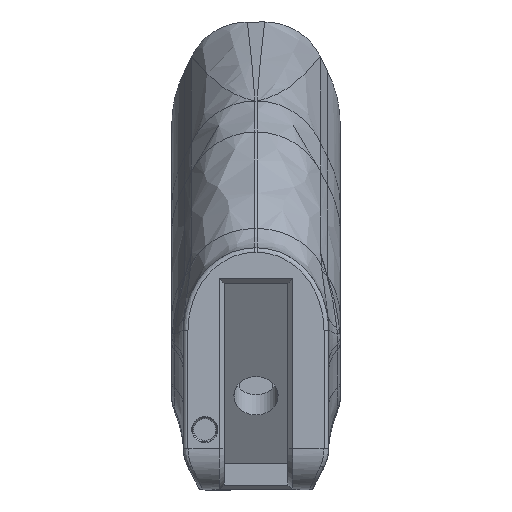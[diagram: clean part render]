
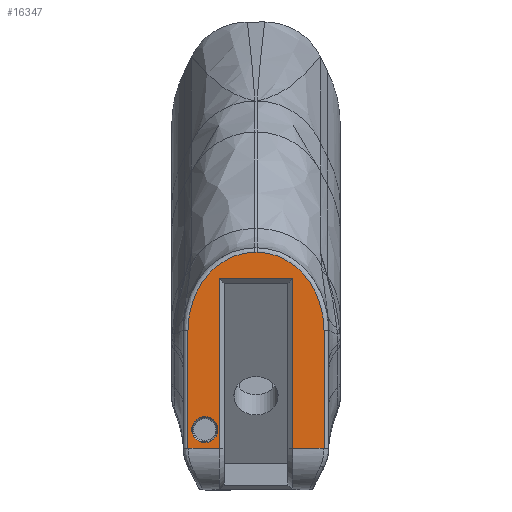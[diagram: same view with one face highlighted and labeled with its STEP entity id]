
A CAD part, top view. The second image highlights one B-rep face of the part: STEP entity #16347.
In plain terms, the highlighted planar face has unit normal (0, 0, 1).
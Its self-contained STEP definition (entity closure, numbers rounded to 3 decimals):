
#970=FACE_BOUND('',#2834,.T.);
#977=CIRCLE('',#17422,2.);
#1773=FACE_OUTER_BOUND('',#2833,.T.);
#2833=EDGE_LOOP('',(#10723,#10724,#10725,#10726,#10727,#10728,#10729,#10730,
#10731,#10732));
#2834=EDGE_LOOP('',(#10733));
#3900=B_SPLINE_CURVE_WITH_KNOTS('',3,(#22767,#22768,#22769,#22770,#22771,
#22772,#22773),.UNSPECIFIED.,.F.,.F.,(4,1,1,1,4),(-1.753,-1.252,
-0.751,-0.25,0.),.UNSPECIFIED.);
#3901=B_SPLINE_CURVE_WITH_KNOTS('',3,(#22788,#22789,#22790,#22791,#22792,
#22793,#22794),.UNSPECIFIED.,.F.,.F.,(4,1,1,1,4),(-1.753,-1.252,
-0.751,-0.25,0.),.UNSPECIFIED.);
#5078=LINE('',#22765,#5718);
#5079=LINE('',#22775,#5719);
#5080=LINE('',#22777,#5720);
#5081=LINE('',#22779,#5721);
#5082=LINE('',#22781,#5722);
#5083=LINE('',#22783,#5723);
#5084=LINE('',#22785,#5724);
#5085=LINE('',#22787,#5725);
#5718=VECTOR('',#18991,10.);
#5719=VECTOR('',#18992,10.);
#5720=VECTOR('',#18993,10.);
#5721=VECTOR('',#18994,10.);
#5722=VECTOR('',#18995,10.);
#5723=VECTOR('',#18996,10.);
#5724=VECTOR('',#18997,10.);
#5725=VECTOR('',#18998,10.);
#6358=VERTEX_POINT('',#22763);
#6359=VERTEX_POINT('',#22764);
#6360=VERTEX_POINT('',#22766);
#6361=VERTEX_POINT('',#22774);
#6362=VERTEX_POINT('',#22776);
#6363=VERTEX_POINT('',#22778);
#6364=VERTEX_POINT('',#22780);
#6365=VERTEX_POINT('',#22782);
#6366=VERTEX_POINT('',#22784);
#6367=VERTEX_POINT('',#22786);
#6368=VERTEX_POINT('',#22795);
#8012=EDGE_CURVE('',#6358,#6359,#5078,.T.);
#8013=EDGE_CURVE('',#6360,#6359,#3900,.T.);
#8014=EDGE_CURVE('',#6361,#6360,#5079,.T.);
#8015=EDGE_CURVE('',#6361,#6362,#5080,.T.);
#8016=EDGE_CURVE('',#6363,#6362,#5081,.T.);
#8017=EDGE_CURVE('',#6363,#6364,#5082,.T.);
#8018=EDGE_CURVE('',#6364,#6365,#5083,.T.);
#8019=EDGE_CURVE('',#6366,#6365,#5084,.T.);
#8020=EDGE_CURVE('',#6366,#6367,#5085,.T.);
#8021=EDGE_CURVE('',#6367,#6358,#3901,.T.);
#8022=EDGE_CURVE('',#6368,#6368,#977,.T.);
#10723=ORIENTED_EDGE('',*,*,#8012,.T.);
#10724=ORIENTED_EDGE('',*,*,#8013,.F.);
#10725=ORIENTED_EDGE('',*,*,#8014,.F.);
#10726=ORIENTED_EDGE('',*,*,#8015,.T.);
#10727=ORIENTED_EDGE('',*,*,#8016,.F.);
#10728=ORIENTED_EDGE('',*,*,#8017,.T.);
#10729=ORIENTED_EDGE('',*,*,#8018,.T.);
#10730=ORIENTED_EDGE('',*,*,#8019,.F.);
#10731=ORIENTED_EDGE('',*,*,#8020,.T.);
#10732=ORIENTED_EDGE('',*,*,#8021,.T.);
#10733=ORIENTED_EDGE('',*,*,#8022,.F.);
#16145=PLANE('',#17421);
#16347=ADVANCED_FACE('',(#1773,#970),#16145,.T.);
#17421=AXIS2_PLACEMENT_3D('',#22762,#18989,#18990);
#17422=AXIS2_PLACEMENT_3D('',#22796,#18999,#19000);
#18989=DIRECTION('center_axis',(0.,0.,
1.));
#18990=DIRECTION('ref_axis',(0.,-1.,0.));
#18991=DIRECTION('',(-1.,0.,0.));
#18992=DIRECTION('',(0.,1.,0.));
#18993=DIRECTION('',(1.,0.,0.));
#18994=DIRECTION('',(0.,-1.,0.));
#18995=DIRECTION('',(1.,0.,0.));
#18996=DIRECTION('',(0.,-1.,0.));
#18997=DIRECTION('',(-1.,0.,0.));
#18998=DIRECTION('',(0.,1.,0.));
#18999=DIRECTION('center_axis',(0.,0.,
1.));
#19000=DIRECTION('ref_axis',(1.,0.,0.));
#22762=CARTESIAN_POINT('Origin',(-5.201,-117.088,-9.218));
#22763=CARTESIAN_POINT('',(-0.163,-117.788,-9.218));
#22764=CARTESIAN_POINT('',(-0.49,-117.788,-9.218));
#22765=CARTESIAN_POINT('',(2.029,-117.788,-9.218));
#22766=CARTESIAN_POINT('',(-10.79,-129.779,-9.218));
#22767=CARTESIAN_POINT('Ctrl Pts',(-10.79,-129.779,
-9.218));
#22768=CARTESIAN_POINT('Ctrl Pts',(-10.79,-128.11,
-9.218));
#22769=CARTESIAN_POINT('Ctrl Pts',(-10.19,-124.771,
-9.218));
#22770=CARTESIAN_POINT('Ctrl Pts',(-7.491,-120.424,
-9.218));
#22771=CARTESIAN_POINT('Ctrl Pts',(-3.836,-118.144,
-9.218));
#22772=CARTESIAN_POINT('Ctrl Pts',(-1.325,-117.788,
-9.218));
#22773=CARTESIAN_POINT('Ctrl Pts',(-0.49,-117.788,
-9.218));
#22774=CARTESIAN_POINT('',(-10.79,-147.932,-9.218));
#22775=CARTESIAN_POINT('',(-10.79,-44.832,-9.218));
#22776=CARTESIAN_POINT('',(-5.991,-147.932,-9.218));
#22777=CARTESIAN_POINT('',(4.548,-147.932,-9.218));
#22778=CARTESIAN_POINT('',(-5.991,-121.782,-9.218));
#22779=CARTESIAN_POINT('',(-5.991,-119.083,-9.218));
#22780=CARTESIAN_POINT('',(5.338,-121.782,-9.218));
#22781=CARTESIAN_POINT('',(-0.418,-121.782,-9.218));
#22782=CARTESIAN_POINT('',(5.338,-147.932,-9.218));
#22783=CARTESIAN_POINT('',(5.338,-119.083,-9.218));
#22784=CARTESIAN_POINT('',(10.137,-147.932,-9.218));
#22785=CARTESIAN_POINT('',(-5.201,-147.932,-9.218));
#22786=CARTESIAN_POINT('',(10.137,-129.779,-9.218));
#22787=CARTESIAN_POINT('',(10.137,-44.832,-9.218));
#22788=CARTESIAN_POINT('Ctrl Pts',(10.137,-129.779,-9.218));
#22789=CARTESIAN_POINT('Ctrl Pts',(10.137,-128.11,-9.218));
#22790=CARTESIAN_POINT('Ctrl Pts',(9.537,-124.771,-9.218));
#22791=CARTESIAN_POINT('Ctrl Pts',(6.838,-120.424,-9.218));
#22792=CARTESIAN_POINT('Ctrl Pts',(3.183,-118.144,-9.218));
#22793=CARTESIAN_POINT('Ctrl Pts',(0.672,-117.788,-9.218));
#22794=CARTESIAN_POINT('Ctrl Pts',(-0.163,-117.788,
-9.218));
#22795=CARTESIAN_POINT('',(-10.203,-145.037,-9.218));
#22796=CARTESIAN_POINT('Origin',(-8.203,-145.037,-9.218));
